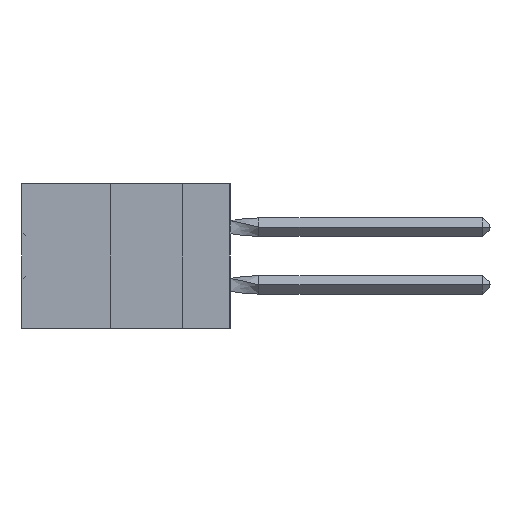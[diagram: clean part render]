
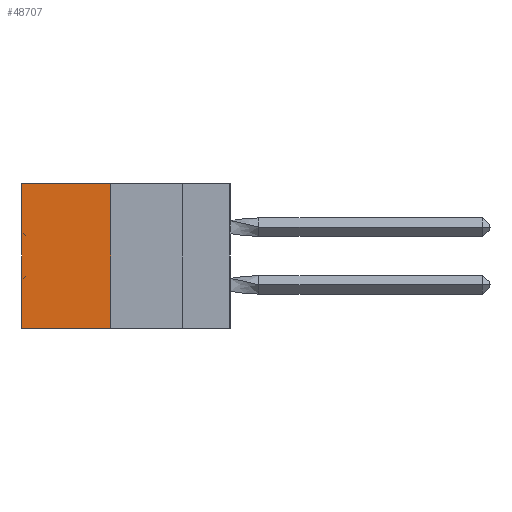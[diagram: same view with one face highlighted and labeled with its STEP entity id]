
A CAD part, left-side view. The second image highlights one B-rep face of the part: STEP entity #48707.
In plain terms, the highlighted planar face has unit normal (-1, 0, 0).
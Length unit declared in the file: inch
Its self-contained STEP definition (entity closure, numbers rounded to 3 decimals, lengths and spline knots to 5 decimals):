
#588 = VERTEX_POINT ( 'NONE', #47476 ) ;
#5529 = ORIENTED_EDGE ( 'NONE', *, *, #48178, .F. ) ;
#6782 = EDGE_CURVE ( 'NONE', #46812, #588, #50016, .T. ) ;
#8125 = ORIENTED_EDGE ( 'NONE', *, *, #52951, .T. ) ;
#9328 = CARTESIAN_POINT ( 'NONE',  ( 0.305, 0.413, -0.5 ) ) ;
#11307 = ORIENTED_EDGE ( 'NONE', *, *, #6782, .T. ) ;
#14279 = LINE ( 'NONE', #35850, #34589 ) ;
#14524 = FACE_OUTER_BOUND ( 'NONE', #58037, .T. ) ;
#14878 = VERTEX_POINT ( 'NONE', #9328 ) ;
#16447 = PLANE ( 'NONE',  #54808 ) ;
#18070 = VERTEX_POINT ( 'NONE', #38448 ) ;
#19928 = CARTESIAN_POINT ( 'NONE',  ( 0.305, 0.72, 0. ) ) ;
#24963 = EDGE_CURVE ( 'NONE', #14878, #588, #35158, .T. ) ;
#25103 = CARTESIAN_POINT ( 'NONE',  ( 0.305, 0.413, -0.5 ) ) ;
#26874 = VECTOR ( 'NONE', #38602, 39.37008 ) ;
#31920 = ORIENTED_EDGE ( 'NONE', *, *, #24963, .F. ) ;
#34116 = DIRECTION ( 'NONE',  ( 0., 0., -1. ) ) ;
#34302 = DIRECTION ( 'NONE',  ( 1., 0., 0. ) ) ;
#34589 = VECTOR ( 'NONE', #57602, 39.37008 ) ;
#35158 = LINE ( 'NONE', #35273, #45681 ) ;
#35273 = CARTESIAN_POINT ( 'NONE',  ( 0.305, 0.413, -0.5 ) ) ;
#35377 = DIRECTION ( 'NONE',  ( 0., 0., -1. ) ) ;
#35469 = DIRECTION ( 'NONE',  ( 0., 1., 0. ) ) ;
#35850 = CARTESIAN_POINT ( 'NONE',  ( 0.305, 0.413, 0. ) ) ;
#38448 = CARTESIAN_POINT ( 'NONE',  ( 0.305, 0.413, 0. ) ) ;
#38602 = DIRECTION ( 'NONE',  ( 0., 0., -1. ) ) ;
#40059 = CARTESIAN_POINT ( 'NONE',  ( 0.305, 0.72, -0.5 ) ) ;
#40853 = LINE ( 'NONE', #52516, #26874 ) ;
#45681 = VECTOR ( 'NONE', #35469, 39.37008 ) ;
#46812 = VERTEX_POINT ( 'NONE', #19928 ) ;
#47476 = CARTESIAN_POINT ( 'NONE',  ( 0.305, 0.72, -0.5 ) ) ;
#48178 = EDGE_CURVE ( 'NONE', #18070, #14878, #40853, .T. ) ;
#48707 = ADVANCED_FACE ( 'NONE', ( #14524 ), #16447, .F. ) ;
#50016 = LINE ( 'NONE', #40059, #52847 ) ;
#52516 = CARTESIAN_POINT ( 'NONE',  ( 0.305, 0.413, -0.5 ) ) ;
#52847 = VECTOR ( 'NONE', #35377, 39.37008 ) ;
#52951 = EDGE_CURVE ( 'NONE', #18070, #46812, #14279, .T. ) ;
#54808 = AXIS2_PLACEMENT_3D ( 'NONE', #25103, #34302, #34116 ) ;
#57602 = DIRECTION ( 'NONE',  ( 0., 1., 0. ) ) ;
#58037 = EDGE_LOOP ( 'NONE', ( #11307, #31920, #5529, #8125 ) ) ;
